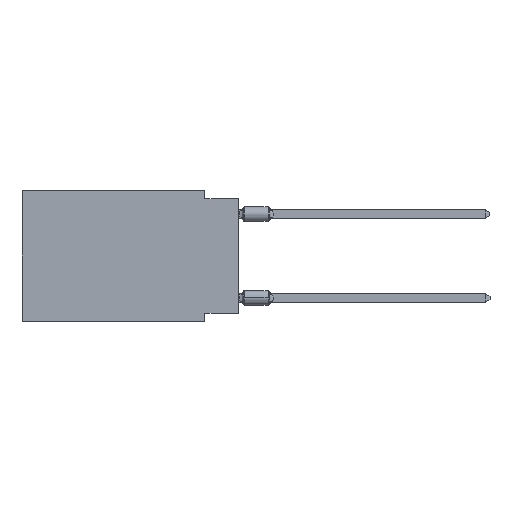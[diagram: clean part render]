
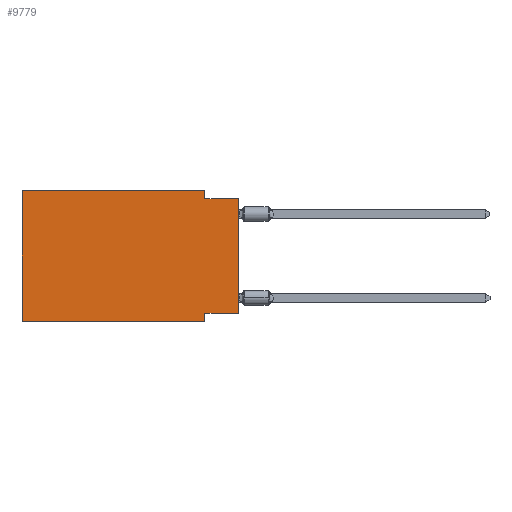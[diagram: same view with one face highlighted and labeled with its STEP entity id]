
A CAD part, left-side view. The second image highlights one B-rep face of the part: STEP entity #9779.
In plain terms, the highlighted planar face has unit normal (-1, 0, 0).
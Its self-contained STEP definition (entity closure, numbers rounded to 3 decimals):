
#227 = CARTESIAN_POINT ( 'NONE',  ( 0., 16.383, -9.906 ) ) ;
#467 = CARTESIAN_POINT ( 'NONE',  ( 0., 2.54, -0.635 ) ) ;
#651 = VECTOR ( 'NONE', #12828, 1000. ) ;
#1517 = LINE ( 'NONE', #15787, #9634 ) ;
#2666 = PLANE ( 'NONE',  #5473 ) ;
#2667 = VERTEX_POINT ( 'NONE', #13011 ) ;
#2687 = DIRECTION ( 'NONE',  ( 0., 0., -1. ) ) ;
#2932 = DIRECTION ( 'NONE',  ( 0., -1., 0. ) ) ;
#3484 = CARTESIAN_POINT ( 'NONE',  ( 0., 0., -0.635 ) ) ;
#3766 = VERTEX_POINT ( 'NONE', #3484 ) ;
#3956 = VECTOR ( 'NONE', #2687, 1000. ) ;
#4820 = CARTESIAN_POINT ( 'NONE',  ( 0., 2.54, -9.906 ) ) ;
#5056 = ORIENTED_EDGE ( 'NONE', *, *, #17188, .F. ) ;
#5085 = ORIENTED_EDGE ( 'NONE', *, *, #9200, .T. ) ;
#5314 = VECTOR ( 'NONE', #5484, 1000. ) ;
#5473 = AXIS2_PLACEMENT_3D ( 'NONE', #15804, #9777, #7178 ) ;
#5484 = DIRECTION ( 'NONE',  ( 0., 1., 0. ) ) ;
#5562 = CARTESIAN_POINT ( 'NONE',  ( 0., 16.383, 0. ) ) ;
#5913 = VERTEX_POINT ( 'NONE', #4820 ) ;
#6350 = DIRECTION ( 'NONE',  ( 0., 0., 1. ) ) ;
#6496 = EDGE_LOOP ( 'NONE', ( #13983, #13757, #11439, #9266, #17852, #5085, #5056, #15322 ) ) ;
#7131 = LINE ( 'NONE', #16987, #651 ) ;
#7178 = DIRECTION ( 'NONE',  ( 0., 0., -1. ) ) ;
#7438 = CARTESIAN_POINT ( 'NONE',  ( 0., 0., -9.271 ) ) ;
#7985 = VERTEX_POINT ( 'NONE', #467 ) ;
#8198 = LINE ( 'NONE', #9678, #17143 ) ;
#8912 = VECTOR ( 'NONE', #18537, 1000. ) ;
#9105 = EDGE_CURVE ( 'NONE', #15641, #13578, #11106, .T. ) ;
#9200 = EDGE_CURVE ( 'NONE', #9227, #5913, #14400, .T. ) ;
#9227 = VERTEX_POINT ( 'NONE', #227 ) ;
#9266 = ORIENTED_EDGE ( 'NONE', *, *, #15170, .F. ) ;
#9601 = EDGE_CURVE ( 'NONE', #7985, #3766, #1517, .T. ) ;
#9602 = LINE ( 'NONE', #13473, #14801 ) ;
#9634 = VECTOR ( 'NONE', #2932, 1000. ) ;
#9678 = CARTESIAN_POINT ( 'NONE',  ( 0., 0., 0. ) ) ;
#9777 = DIRECTION ( 'NONE',  ( 1., 0., 0. ) ) ;
#9779 = ADVANCED_FACE ( 'NONE', ( #17315 ), #2666, .F. ) ;
#9961 = CARTESIAN_POINT ( 'NONE',  ( 0., 16.383, 0. ) ) ;
#11106 = LINE ( 'NONE', #12417, #5314 ) ;
#11439 = ORIENTED_EDGE ( 'NONE', *, *, #12308, .F. ) ;
#11800 = VECTOR ( 'NONE', #14388, 1000. ) ;
#12308 = EDGE_CURVE ( 'NONE', #2667, #7985, #12715, .T. ) ;
#12417 = CARTESIAN_POINT ( 'NONE',  ( 0., 0., -9.271 ) ) ;
#12598 = EDGE_CURVE ( 'NONE', #15641, #3766, #8198, .T. ) ;
#12715 = LINE ( 'NONE', #18459, #3956 ) ;
#12828 = DIRECTION ( 'NONE',  ( 0., 0., -1. ) ) ;
#12995 = CARTESIAN_POINT ( 'NONE',  ( 0., 2.54, -9.271 ) ) ;
#13011 = CARTESIAN_POINT ( 'NONE',  ( 0., 2.54, 0. ) ) ;
#13166 = VERTEX_POINT ( 'NONE', #5562 ) ;
#13473 = CARTESIAN_POINT ( 'NONE',  ( 0., 16.383, 0. ) ) ;
#13578 = VERTEX_POINT ( 'NONE', #12995 ) ;
#13757 = ORIENTED_EDGE ( 'NONE', *, *, #9601, .F. ) ;
#13983 = ORIENTED_EDGE ( 'NONE', *, *, #12598, .T. ) ;
#14388 = DIRECTION ( 'NONE',  ( 0., -1., 0. ) ) ;
#14400 = LINE ( 'NONE', #15618, #8912 ) ;
#14801 = VECTOR ( 'NONE', #6350, 1000. ) ;
#15170 = EDGE_CURVE ( 'NONE', #13166, #2667, #17114, .T. ) ;
#15261 = DIRECTION ( 'NONE',  ( 0., 0., 1. ) ) ;
#15322 = ORIENTED_EDGE ( 'NONE', *, *, #9105, .F. ) ;
#15618 = CARTESIAN_POINT ( 'NONE',  ( 0., 16.383, -9.906 ) ) ;
#15641 = VERTEX_POINT ( 'NONE', #7438 ) ;
#15787 = CARTESIAN_POINT ( 'NONE',  ( 0., 0., -0.635 ) ) ;
#15804 = CARTESIAN_POINT ( 'NONE',  ( 0., 16.383, 0. ) ) ;
#16263 = EDGE_CURVE ( 'NONE', #9227, #13166, #9602, .T. ) ;
#16987 = CARTESIAN_POINT ( 'NONE',  ( 0., 2.54, -9.906 ) ) ;
#17114 = LINE ( 'NONE', #9961, #11800 ) ;
#17143 = VECTOR ( 'NONE', #15261, 1000. ) ;
#17188 = EDGE_CURVE ( 'NONE', #13578, #5913, #7131, .T. ) ;
#17315 = FACE_OUTER_BOUND ( 'NONE', #6496, .T. ) ;
#17852 = ORIENTED_EDGE ( 'NONE', *, *, #16263, .F. ) ;
#18459 = CARTESIAN_POINT ( 'NONE',  ( 0., 2.54, 0. ) ) ;
#18537 = DIRECTION ( 'NONE',  ( 0., -1., 0. ) ) ;
